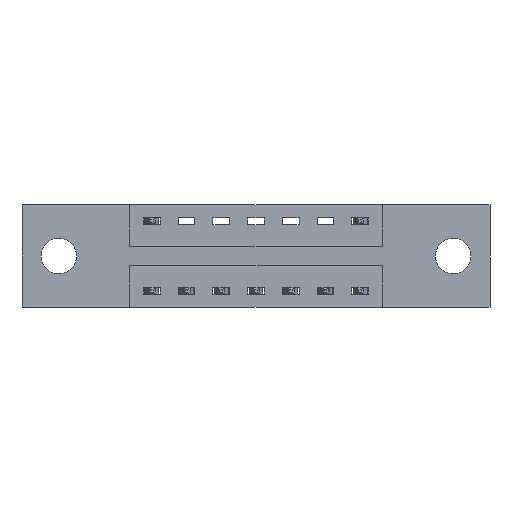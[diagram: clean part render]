
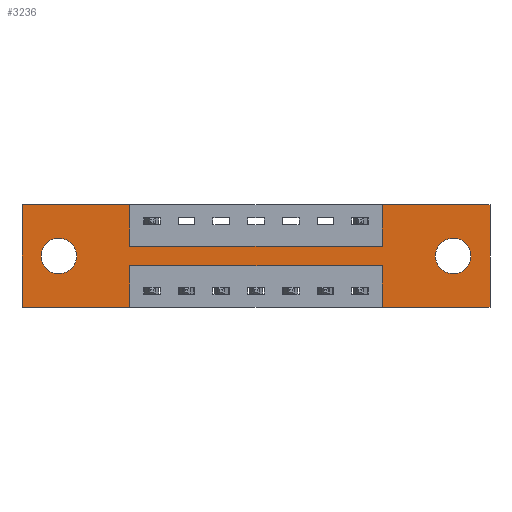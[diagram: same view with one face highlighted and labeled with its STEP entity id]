
A CAD part, front view. The second image highlights one B-rep face of the part: STEP entity #3236.
In plain terms, the highlighted planar face has unit normal (0, -1, 0).
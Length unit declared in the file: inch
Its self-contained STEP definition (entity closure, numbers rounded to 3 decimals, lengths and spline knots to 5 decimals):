
#86 = CARTESIAN_POINT ( 'NONE',  ( 1.2975, 0., -0.22 ) ) ;
#99 = EDGE_LOOP ( 'NONE', ( #3499, #3255 ) ) ;
#147 = EDGE_CURVE ( 'NONE', #2783, #7960, #6540, .T. ) ;
#179 = DIRECTION ( 'NONE',  ( 0., 0., 1. ) ) ;
#193 = ORIENTED_EDGE ( 'NONE', *, *, #572, .T. ) ;
#223 = DIRECTION ( 'NONE',  ( 0., 1., 0. ) ) ;
#367 = CARTESIAN_POINT ( 'NONE',  ( 1.2975, 0., -0.37 ) ) ;
#547 = EDGE_CURVE ( 'NONE', #3050, #7231, #7496, .T. ) ;
#572 = EDGE_CURVE ( 'NONE', #8431, #6460, #9031, .T. ) ;
#586 = FACE_BOUND ( 'NONE', #99, .T. ) ;
#599 = EDGE_CURVE ( 'NONE', #7960, #2783, #4934, .T. ) ;
#656 = EDGE_CURVE ( 'NONE', #704, #6441, #8214, .T. ) ;
#697 = DIRECTION ( 'NONE',  ( 0., 0., -1. ) ) ;
#704 = VERTEX_POINT ( 'NONE', #4414 ) ;
#712 = EDGE_CURVE ( 'NONE', #7231, #704, #7815, .T. ) ;
#722 = CARTESIAN_POINT ( 'NONE',  ( 0.3875, 0., 0. ) ) ;
#1056 = LINE ( 'NONE', #2689, #8372 ) ;
#1160 = AXIS2_PLACEMENT_3D ( 'NONE', #2774, #7115, #3353 ) ;
#1211 = EDGE_CURVE ( 'NONE', #3840, #6716, #4173, .T. ) ;
#1221 = DIRECTION ( 'NONE',  ( 1., 0., 0. ) ) ;
#1277 = EDGE_CURVE ( 'NONE', #5555, #5814, #8812, .T. ) ;
#1391 = DIRECTION ( 'NONE',  ( 0., 0., -1. ) ) ;
#1395 = LINE ( 'NONE', #8504, #8470 ) ;
#1404 = ORIENTED_EDGE ( 'NONE', *, *, #3611, .F. ) ;
#1432 = CARTESIAN_POINT ( 'NONE',  ( 1.685, 0., 0. ) ) ;
#1463 = EDGE_CURVE ( 'NONE', #8033, #1648, #2969, .T. ) ;
#1593 = CARTESIAN_POINT ( 'NONE',  ( 1.5525, 0., -0.249 ) ) ;
#1648 = VERTEX_POINT ( 'NONE', #4596 ) ;
#1791 = EDGE_LOOP ( 'NONE', ( #3510, #4897, #7980, #2140, #3281, #4884, #2366, #3815, #9079, #7341, #7121, #1404 ) ) ;
#1826 = VECTOR ( 'NONE', #5823, 39.37008 ) ;
#1938 = VECTOR ( 'NONE', #179, 39.37008 ) ;
#1944 = DIRECTION ( 'NONE',  ( -1., 0., 0. ) ) ;
#2068 = EDGE_CURVE ( 'NONE', #8330, #5555, #4583, .T. ) ;
#2114 = CARTESIAN_POINT ( 'NONE',  ( 1.5525, 0., -0.185 ) ) ;
#2140 = ORIENTED_EDGE ( 'NONE', *, *, #4023, .F. ) ;
#2152 = EDGE_CURVE ( 'NONE', #6460, #8431, #8091, .T. ) ;
#2192 = CARTESIAN_POINT ( 'NONE',  ( 0.3875, 0., -0.22 ) ) ;
#2256 = EDGE_CURVE ( 'NONE', #6716, #5813, #7036, .T. ) ;
#2288 = ORIENTED_EDGE ( 'NONE', *, *, #2152, .T. ) ;
#2291 = VECTOR ( 'NONE', #1221, 39.37008 ) ;
#2293 = CARTESIAN_POINT ( 'NONE',  ( 0.3875, 0., -0.37 ) ) ;
#2301 = CARTESIAN_POINT ( 'NONE',  ( 0., 0., 0. ) ) ;
#2346 = AXIS2_PLACEMENT_3D ( 'NONE', #8485, #5020, #697 ) ;
#2366 = ORIENTED_EDGE ( 'NONE', *, *, #7375, .F. ) ;
#2476 = LINE ( 'NONE', #7468, #6016 ) ;
#2608 = CARTESIAN_POINT ( 'NONE',  ( 1.685, 0., 0. ) ) ;
#2648 = CARTESIAN_POINT ( 'NONE',  ( 0.1325, 0., -0.249 ) ) ;
#2689 = CARTESIAN_POINT ( 'NONE',  ( 0., 0., -0.37 ) ) ;
#2720 = VECTOR ( 'NONE', #2940, 39.37008 ) ;
#2774 = CARTESIAN_POINT ( 'NONE',  ( 1.5525, 0., -0.185 ) ) ;
#2783 = VERTEX_POINT ( 'NONE', #2648 ) ;
#2852 = DIRECTION ( 'NONE',  ( 0., 0., -1. ) ) ;
#2932 = PLANE ( 'NONE',  #2346 ) ;
#2940 = DIRECTION ( 'NONE',  ( 1., 0., 0. ) ) ;
#2969 = LINE ( 'NONE', #8490, #2720 ) ;
#3050 = VERTEX_POINT ( 'NONE', #367 ) ;
#3153 = EDGE_LOOP ( 'NONE', ( #193, #2288 ) ) ;
#3170 = AXIS2_PLACEMENT_3D ( 'NONE', #8466, #6600, #7363 ) ;
#3236 = ADVANCED_FACE ( 'NONE', ( #8172, #586, #4448 ), #2932, .T. ) ;
#3255 = ORIENTED_EDGE ( 'NONE', *, *, #147, .T. ) ;
#3281 = ORIENTED_EDGE ( 'NONE', *, *, #2256, .F. ) ;
#3353 = DIRECTION ( 'NONE',  ( 0., 0., -1. ) ) ;
#3499 = ORIENTED_EDGE ( 'NONE', *, *, #599, .T. ) ;
#3510 = ORIENTED_EDGE ( 'NONE', *, *, #656, .F. ) ;
#3611 = EDGE_CURVE ( 'NONE', #6441, #8330, #1056, .T. ) ;
#3683 = CARTESIAN_POINT ( 'NONE',  ( 0., 0., 0. ) ) ;
#3815 = ORIENTED_EDGE ( 'NONE', *, *, #1463, .F. ) ;
#3840 = VERTEX_POINT ( 'NONE', #7773 ) ;
#3850 = CARTESIAN_POINT ( 'NONE',  ( 1.2975, 0., 0. ) ) ;
#4023 = EDGE_CURVE ( 'NONE', #5813, #3050, #1395, .T. ) ;
#4048 = AXIS2_PLACEMENT_3D ( 'NONE', #2114, #7083, #2852 ) ;
#4173 = LINE ( 'NONE', #2301, #2291 ) ;
#4414 = CARTESIAN_POINT ( 'NONE',  ( 0.3875, 0., -0.22 ) ) ;
#4448 = FACE_OUTER_BOUND ( 'NONE', #1791, .T. ) ;
#4495 = VECTOR ( 'NONE', #1391, 39.37008 ) ;
#4540 = EDGE_CURVE ( 'NONE', #5814, #8033, #2476, .T. ) ;
#4552 = CARTESIAN_POINT ( 'NONE',  ( 1.5525, 0., -0.121 ) ) ;
#4583 = LINE ( 'NONE', #4762, #8094 ) ;
#4596 = CARTESIAN_POINT ( 'NONE',  ( 1.2975, 0., -0.15 ) ) ;
#4711 = VECTOR ( 'NONE', #6043, 39.37008 ) ;
#4762 = CARTESIAN_POINT ( 'NONE',  ( 0., 0., 0. ) ) ;
#4862 = DIRECTION ( 'NONE',  ( 0., 0., 1. ) ) ;
#4884 = ORIENTED_EDGE ( 'NONE', *, *, #1211, .F. ) ;
#4897 = ORIENTED_EDGE ( 'NONE', *, *, #712, .F. ) ;
#4914 = DIRECTION ( 'NONE',  ( 1., 0., 0. ) ) ;
#4922 = CARTESIAN_POINT ( 'NONE',  ( 0.1325, 0., -0.121 ) ) ;
#4934 = CIRCLE ( 'NONE', #3170, 0.064 ) ;
#4955 = CARTESIAN_POINT ( 'NONE',  ( 0.3875, 0., -0.15 ) ) ;
#5020 = DIRECTION ( 'NONE',  ( 0., -1., 0. ) ) ;
#5041 = DIRECTION ( 'NONE',  ( 0., 0., -1. ) ) ;
#5045 = CARTESIAN_POINT ( 'NONE',  ( 1.685, 0., -0.37 ) ) ;
#5140 = VECTOR ( 'NONE', #4914, 39.37008 ) ;
#5170 = CARTESIAN_POINT ( 'NONE',  ( 0., 0., -0.37 ) ) ;
#5555 = VERTEX_POINT ( 'NONE', #7449 ) ;
#5713 = AXIS2_PLACEMENT_3D ( 'NONE', #7947, #223, #4862 ) ;
#5813 = VERTEX_POINT ( 'NONE', #5045 ) ;
#5814 = VERTEX_POINT ( 'NONE', #722 ) ;
#5823 = DIRECTION ( 'NONE',  ( 0., 0., 1. ) ) ;
#5968 = LINE ( 'NONE', #3850, #1938 ) ;
#6016 = VECTOR ( 'NONE', #6791, 39.37008 ) ;
#6043 = DIRECTION ( 'NONE',  ( -1., 0., 0. ) ) ;
#6441 = VERTEX_POINT ( 'NONE', #7983 ) ;
#6460 = VERTEX_POINT ( 'NONE', #1593 ) ;
#6540 = CIRCLE ( 'NONE', #5713, 0.064 ) ;
#6600 = DIRECTION ( 'NONE',  ( 0., 1., 0. ) ) ;
#6716 = VERTEX_POINT ( 'NONE', #2608 ) ;
#6791 = DIRECTION ( 'NONE',  ( 0., 0., -1. ) ) ;
#7036 = LINE ( 'NONE', #1432, #8798 ) ;
#7083 = DIRECTION ( 'NONE',  ( 0., 1., 0. ) ) ;
#7115 = DIRECTION ( 'NONE',  ( 0., 1., 0. ) ) ;
#7121 = ORIENTED_EDGE ( 'NONE', *, *, #2068, .F. ) ;
#7231 = VERTEX_POINT ( 'NONE', #86 ) ;
#7341 = ORIENTED_EDGE ( 'NONE', *, *, #1277, .F. ) ;
#7363 = DIRECTION ( 'NONE',  ( 0., 0., 1. ) ) ;
#7375 = EDGE_CURVE ( 'NONE', #1648, #3840, #5968, .T. ) ;
#7449 = CARTESIAN_POINT ( 'NONE',  ( 0., 0., 0. ) ) ;
#7468 = CARTESIAN_POINT ( 'NONE',  ( 0.3875, 0., 0. ) ) ;
#7496 = LINE ( 'NONE', #7694, #1826 ) ;
#7694 = CARTESIAN_POINT ( 'NONE',  ( 1.2975, 0., -0.37 ) ) ;
#7773 = CARTESIAN_POINT ( 'NONE',  ( 1.2975, 0., 0. ) ) ;
#7815 = LINE ( 'NONE', #2192, #4711 ) ;
#7947 = CARTESIAN_POINT ( 'NONE',  ( 0.1325, 0., -0.185 ) ) ;
#7960 = VERTEX_POINT ( 'NONE', #4922 ) ;
#7980 = ORIENTED_EDGE ( 'NONE', *, *, #547, .F. ) ;
#7983 = CARTESIAN_POINT ( 'NONE',  ( 0.3875, 0., -0.37 ) ) ;
#8033 = VERTEX_POINT ( 'NONE', #4955 ) ;
#8091 = CIRCLE ( 'NONE', #4048, 0.064 ) ;
#8094 = VECTOR ( 'NONE', #8247, 39.37008 ) ;
#8172 = FACE_BOUND ( 'NONE', #3153, .T. ) ;
#8214 = LINE ( 'NONE', #2293, #4495 ) ;
#8247 = DIRECTION ( 'NONE',  ( 0., 0., 1. ) ) ;
#8330 = VERTEX_POINT ( 'NONE', #5170 ) ;
#8372 = VECTOR ( 'NONE', #1944, 39.37008 ) ;
#8431 = VERTEX_POINT ( 'NONE', #4552 ) ;
#8466 = CARTESIAN_POINT ( 'NONE',  ( 0.1325, 0., -0.185 ) ) ;
#8470 = VECTOR ( 'NONE', #9159, 39.37008 ) ;
#8485 = CARTESIAN_POINT ( 'NONE',  ( 0., 0., -0.37 ) ) ;
#8490 = CARTESIAN_POINT ( 'NONE',  ( 0.3875, 0., -0.15 ) ) ;
#8504 = CARTESIAN_POINT ( 'NONE',  ( 0., 0., -0.37 ) ) ;
#8798 = VECTOR ( 'NONE', #5041, 39.37008 ) ;
#8812 = LINE ( 'NONE', #3683, #5140 ) ;
#9031 = CIRCLE ( 'NONE', #1160, 0.064 ) ;
#9079 = ORIENTED_EDGE ( 'NONE', *, *, #4540, .F. ) ;
#9159 = DIRECTION ( 'NONE',  ( -1., 0., 0. ) ) ;
